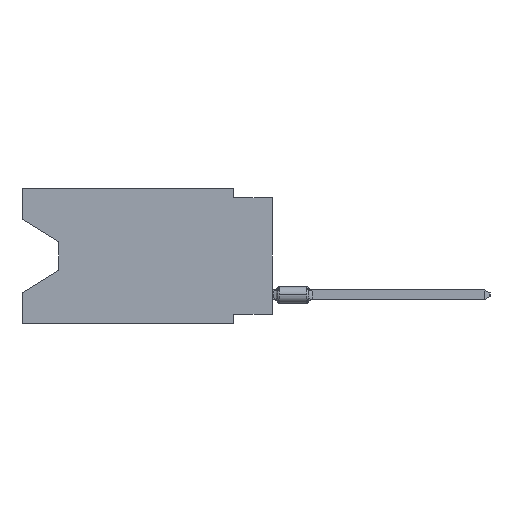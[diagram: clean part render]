
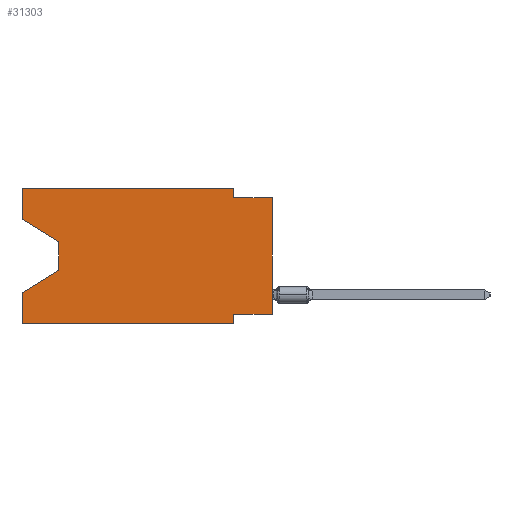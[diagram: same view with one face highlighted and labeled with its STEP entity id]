
A CAD part, left-side view. The second image highlights one B-rep face of the part: STEP entity #31303.
In plain terms, the highlighted planar face has unit normal (-1, 0, 0).
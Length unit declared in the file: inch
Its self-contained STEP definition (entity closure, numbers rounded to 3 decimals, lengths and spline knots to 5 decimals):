
#454 = LINE ( 'NONE', #31232, #39732 ) ;
#1007 = EDGE_CURVE ( 'NONE', #17435, #22656, #38868, .T. ) ;
#1022 = VECTOR ( 'NONE', #24024, 39.37008 ) ;
#1313 = CARTESIAN_POINT ( 'NONE',  ( 0., 0.55, -0.138 ) ) ;
#1575 = VERTEX_POINT ( 'NONE', #15754 ) ;
#1895 = CARTESIAN_POINT ( 'NONE',  ( 0., 0.645, 0. ) ) ;
#1917 = DIRECTION ( 'NONE',  ( 0., -1., 0. ) ) ;
#2125 = ORIENTED_EDGE ( 'NONE', *, *, #19465, .T. ) ;
#2529 = VECTOR ( 'NONE', #37432, 39.37008 ) ;
#2534 = CARTESIAN_POINT ( 'NONE',  ( 0., 0., -0.325 ) ) ;
#3376 = VERTEX_POINT ( 'NONE', #9214 ) ;
#3564 = ORIENTED_EDGE ( 'NONE', *, *, #16571, .F. ) ;
#3975 = EDGE_CURVE ( 'NONE', #9996, #17435, #4904, .T. ) ;
#4206 = LINE ( 'NONE', #25354, #2529 ) ;
#4724 = VERTEX_POINT ( 'NONE', #12920 ) ;
#4904 = LINE ( 'NONE', #37932, #18846 ) ;
#5289 = DIRECTION ( 'NONE',  ( 0., 0., -1. ) ) ;
#5466 = ORIENTED_EDGE ( 'NONE', *, *, #1007, .F. ) ;
#5556 = DIRECTION ( 'NONE',  ( 0., 0., -1. ) ) ;
#5559 = ORIENTED_EDGE ( 'NONE', *, *, #7570, .T. ) ;
#5773 = VECTOR ( 'NONE', #29883, 39.37008 ) ;
#5991 = DIRECTION ( 'NONE',  ( 0., -1., 0. ) ) ;
#7570 = EDGE_CURVE ( 'NONE', #1575, #3376, #454, .T. ) ;
#8158 = CARTESIAN_POINT ( 'NONE',  ( 0., 0.645, 0. ) ) ;
#8389 = CARTESIAN_POINT ( 'NONE',  ( 0., 0.55, -0.138 ) ) ;
#9214 = CARTESIAN_POINT ( 'NONE',  ( 0., 0.645, -0.26975 ) ) ;
#9996 = VERTEX_POINT ( 'NONE', #2534 ) ;
#10374 = DIRECTION ( 'NONE',  ( 0., 1., 0. ) ) ;
#10677 = ORIENTED_EDGE ( 'NONE', *, *, #25452, .T. ) ;
#11113 = CARTESIAN_POINT ( 'NONE',  ( 0., 0.645, -0.08025 ) ) ;
#11492 = CARTESIAN_POINT ( 'NONE',  ( 0., 0.645, -0.35 ) ) ;
#12431 = EDGE_CURVE ( 'NONE', #4724, #19192, #26838, .T. ) ;
#12920 = CARTESIAN_POINT ( 'NONE',  ( 0., 0.645, 0. ) ) ;
#13888 = VECTOR ( 'NONE', #23786, 39.37008 ) ;
#14164 = VECTOR ( 'NONE', #5991, 39.37008 ) ;
#14202 = LINE ( 'NONE', #35511, #38567 ) ;
#14705 = CARTESIAN_POINT ( 'NONE',  ( 0., 0., -0.025 ) ) ;
#15317 = VERTEX_POINT ( 'NONE', #14705 ) ;
#15318 = ORIENTED_EDGE ( 'NONE', *, *, #23653, .F. ) ;
#15754 = CARTESIAN_POINT ( 'NONE',  ( 0., 0.55, -0.212 ) ) ;
#16571 = EDGE_CURVE ( 'NONE', #31024, #15317, #27128, .T. ) ;
#17264 = ORIENTED_EDGE ( 'NONE', *, *, #36449, .T. ) ;
#17299 = ORIENTED_EDGE ( 'NONE', *, *, #24189, .F. ) ;
#17435 = VERTEX_POINT ( 'NONE', #24707 ) ;
#17959 = DIRECTION ( 'NONE',  ( 1., 0., 0. ) ) ;
#18056 = CARTESIAN_POINT ( 'NONE',  ( 0., 0., -0.025 ) ) ;
#18366 = LINE ( 'NONE', #24431, #1022 ) ;
#18846 = VECTOR ( 'NONE', #10374, 39.37008 ) ;
#19192 = VERTEX_POINT ( 'NONE', #36306 ) ;
#19465 = EDGE_CURVE ( 'NONE', #21252, #20695, #25642, .T. ) ;
#20695 = VERTEX_POINT ( 'NONE', #1313 ) ;
#21011 = ORIENTED_EDGE ( 'NONE', *, *, #3975, .F. ) ;
#21252 = VERTEX_POINT ( 'NONE', #11113 ) ;
#22656 = VERTEX_POINT ( 'NONE', #26596 ) ;
#22858 = VECTOR ( 'NONE', #5289, 39.37008 ) ;
#23379 = VECTOR ( 'NONE', #26220, 39.37008 ) ;
#23653 = EDGE_CURVE ( 'NONE', #19192, #31024, #18366, .T. ) ;
#23786 = DIRECTION ( 'NONE',  ( 0., 0., 1. ) ) ;
#24024 = DIRECTION ( 'NONE',  ( 0., 0., -1. ) ) ;
#24189 = EDGE_CURVE ( 'NONE', #38521, #3376, #30008, .T. ) ;
#24431 = CARTESIAN_POINT ( 'NONE',  ( 0., 0.1, 0. ) ) ;
#24707 = CARTESIAN_POINT ( 'NONE',  ( 0., 0.1, -0.325 ) ) ;
#25155 = EDGE_LOOP ( 'NONE', ( #2125, #10677, #5559, #17299, #17264, #5466, #21011, #35182, #3564, #15318, #36440, #28613 ) ) ;
#25354 = CARTESIAN_POINT ( 'NONE',  ( 0., 0., 0. ) ) ;
#25452 = EDGE_CURVE ( 'NONE', #20695, #1575, #33516, .T. ) ;
#25642 = LINE ( 'NONE', #31664, #23379 ) ;
#26220 = DIRECTION ( 'NONE',  ( 0., -0.855, -0.519 ) ) ;
#26236 = DIRECTION ( 'NONE',  ( 0., -1., 0. ) ) ;
#26596 = CARTESIAN_POINT ( 'NONE',  ( 0., 0.1, -0.35 ) ) ;
#26829 = FACE_OUTER_BOUND ( 'NONE', #25155, .T. ) ;
#26838 = LINE ( 'NONE', #1895, #38355 ) ;
#27128 = LINE ( 'NONE', #18056, #14164 ) ;
#28299 = CARTESIAN_POINT ( 'NONE',  ( 0., 0.1, -0.025 ) ) ;
#28613 = ORIENTED_EDGE ( 'NONE', *, *, #37720, .F. ) ;
#29883 = DIRECTION ( 'NONE',  ( 0., 0., 1. ) ) ;
#30008 = LINE ( 'NONE', #33218, #13888 ) ;
#30039 = PLANE ( 'NONE',  #34049 ) ;
#31024 = VERTEX_POINT ( 'NONE', #28299 ) ;
#31232 = CARTESIAN_POINT ( 'NONE',  ( 0., 0.55, -0.212 ) ) ;
#31303 = ADVANCED_FACE ( 'NONE', ( #26829 ), #30039, .F. ) ;
#31664 = CARTESIAN_POINT ( 'NONE',  ( 0., 0.645, -0.08025 ) ) ;
#31897 = VECTOR ( 'NONE', #5556, 39.37008 ) ;
#33218 = CARTESIAN_POINT ( 'NONE',  ( 0., 0.645, 0. ) ) ;
#33516 = LINE ( 'NONE', #8389, #31897 ) ;
#34049 = AXIS2_PLACEMENT_3D ( 'NONE', #36267, #17959, #39485 ) ;
#35182 = ORIENTED_EDGE ( 'NONE', *, *, #35710, .T. ) ;
#35511 = CARTESIAN_POINT ( 'NONE',  ( 0., 0.645, -0.35 ) ) ;
#35710 = EDGE_CURVE ( 'NONE', #9996, #15317, #4206, .T. ) ;
#35854 = CARTESIAN_POINT ( 'NONE',  ( 0., 0.1, -0.35 ) ) ;
#36267 = CARTESIAN_POINT ( 'NONE',  ( 0., 0.645, 0. ) ) ;
#36306 = CARTESIAN_POINT ( 'NONE',  ( 0., 0.1, 0. ) ) ;
#36440 = ORIENTED_EDGE ( 'NONE', *, *, #12431, .F. ) ;
#36449 = EDGE_CURVE ( 'NONE', #38521, #22656, #14202, .T. ) ;
#37284 = DIRECTION ( 'NONE',  ( 0., 0.855, -0.519 ) ) ;
#37432 = DIRECTION ( 'NONE',  ( 0., 0., 1. ) ) ;
#37720 = EDGE_CURVE ( 'NONE', #21252, #4724, #38932, .T. ) ;
#37932 = CARTESIAN_POINT ( 'NONE',  ( 0., 0., -0.325 ) ) ;
#38355 = VECTOR ( 'NONE', #26236, 39.37008 ) ;
#38521 = VERTEX_POINT ( 'NONE', #11492 ) ;
#38567 = VECTOR ( 'NONE', #1917, 39.37008 ) ;
#38868 = LINE ( 'NONE', #35854, #22858 ) ;
#38932 = LINE ( 'NONE', #8158, #5773 ) ;
#39485 = DIRECTION ( 'NONE',  ( 0., 0., -1. ) ) ;
#39732 = VECTOR ( 'NONE', #37284, 39.37008 ) ;
